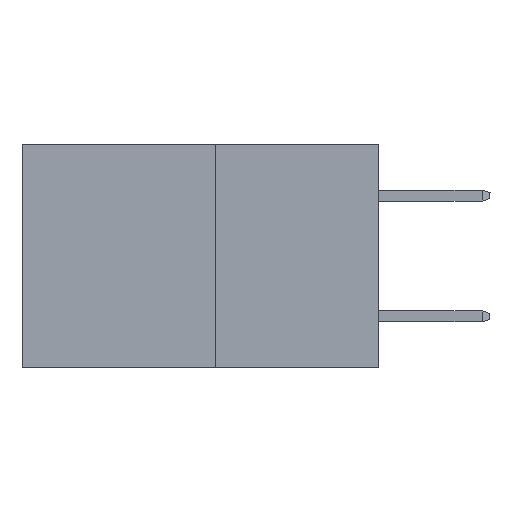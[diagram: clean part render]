
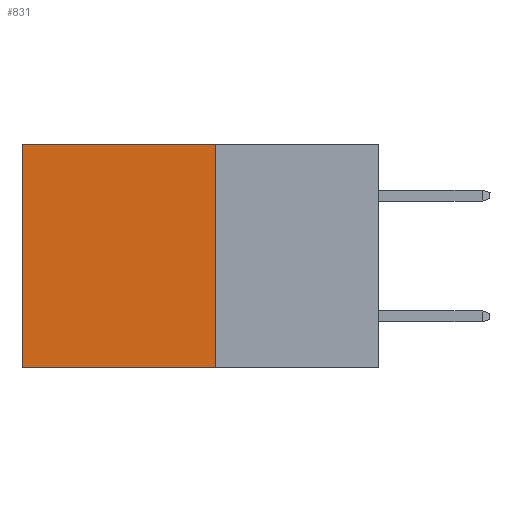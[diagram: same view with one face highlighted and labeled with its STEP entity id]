
A CAD part, left-side view. The second image highlights one B-rep face of the part: STEP entity #831.
In plain terms, the highlighted planar face has unit normal (-1, 0, 0).
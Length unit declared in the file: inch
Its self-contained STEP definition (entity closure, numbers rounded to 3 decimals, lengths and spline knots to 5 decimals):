
#483 = LINE ( 'NONE', #6013, #11288 ) ;
#831 = ADVANCED_FACE ( 'NONE', ( #17000 ), #17983, .F. ) ;
#847 = EDGE_CURVE ( 'NONE', #4671, #14925, #5895, .T. ) ;
#1681 = EDGE_CURVE ( 'NONE', #14925, #12356, #483, .T. ) ;
#1943 = EDGE_LOOP ( 'NONE', ( #9536, #9299, #3865, #12966 ) ) ;
#2103 = CARTESIAN_POINT ( 'NONE',  ( 0.277, 0.27, -0.37 ) ) ;
#2303 = VECTOR ( 'NONE', #10813, 39.37008 ) ;
#3606 = VERTEX_POINT ( 'NONE', #2103 ) ;
#3641 = CARTESIAN_POINT ( 'NONE',  ( 0.277, 0.27, -0.37 ) ) ;
#3865 = ORIENTED_EDGE ( 'NONE', *, *, #4204, .F. ) ;
#4204 = EDGE_CURVE ( 'NONE', #4671, #3606, #6072, .T. ) ;
#4213 = CARTESIAN_POINT ( 'NONE',  ( 0.277, 0.59, 0. ) ) ;
#4671 = VERTEX_POINT ( 'NONE', #9974 ) ;
#5895 = LINE ( 'NONE', #12993, #9631 ) ;
#6013 = CARTESIAN_POINT ( 'NONE',  ( 0.277, 0.59, -0.37 ) ) ;
#6072 = LINE ( 'NONE', #3641, #2303 ) ;
#7365 = DIRECTION ( 'NONE',  ( 1., 0., 0. ) ) ;
#8486 = EDGE_CURVE ( 'NONE', #3606, #12356, #15465, .T. ) ;
#9299 = ORIENTED_EDGE ( 'NONE', *, *, #8486, .F. ) ;
#9536 = ORIENTED_EDGE ( 'NONE', *, *, #1681, .T. ) ;
#9631 = VECTOR ( 'NONE', #14251, 39.37008 ) ;
#9974 = CARTESIAN_POINT ( 'NONE',  ( 0.277, 0.27, 0. ) ) ;
#10033 = CARTESIAN_POINT ( 'NONE',  ( 0.277, 0.59, -0.37 ) ) ;
#10813 = DIRECTION ( 'NONE',  ( 0., 0., -1. ) ) ;
#11288 = VECTOR ( 'NONE', #17395, 39.37008 ) ;
#11347 = VECTOR ( 'NONE', #12811, 39.37008 ) ;
#11617 = AXIS2_PLACEMENT_3D ( 'NONE', #12572, #7365, #14062 ) ;
#12356 = VERTEX_POINT ( 'NONE', #10033 ) ;
#12572 = CARTESIAN_POINT ( 'NONE',  ( 0.277, 0.27, -0.37 ) ) ;
#12811 = DIRECTION ( 'NONE',  ( 0., 1., 0. ) ) ;
#12966 = ORIENTED_EDGE ( 'NONE', *, *, #847, .T. ) ;
#12993 = CARTESIAN_POINT ( 'NONE',  ( 0.277, 0.27, 0. ) ) ;
#12996 = CARTESIAN_POINT ( 'NONE',  ( 0.277, 0.27, -0.37 ) ) ;
#14062 = DIRECTION ( 'NONE',  ( 0., 0., -1. ) ) ;
#14251 = DIRECTION ( 'NONE',  ( 0., 1., 0. ) ) ;
#14925 = VERTEX_POINT ( 'NONE', #4213 ) ;
#15465 = LINE ( 'NONE', #12996, #11347 ) ;
#17000 = FACE_OUTER_BOUND ( 'NONE', #1943, .T. ) ;
#17395 = DIRECTION ( 'NONE',  ( 0., 0., -1. ) ) ;
#17983 = PLANE ( 'NONE',  #11617 ) ;
